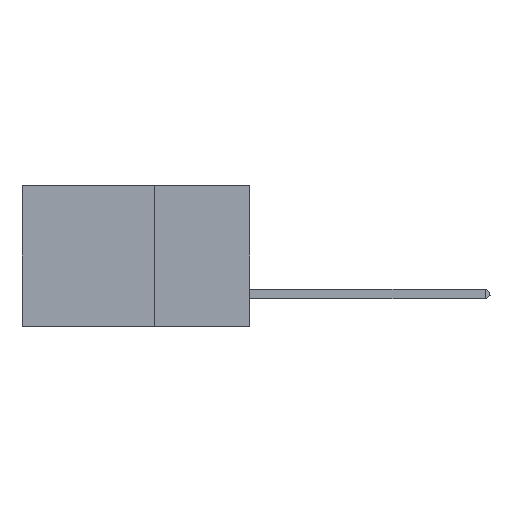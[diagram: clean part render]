
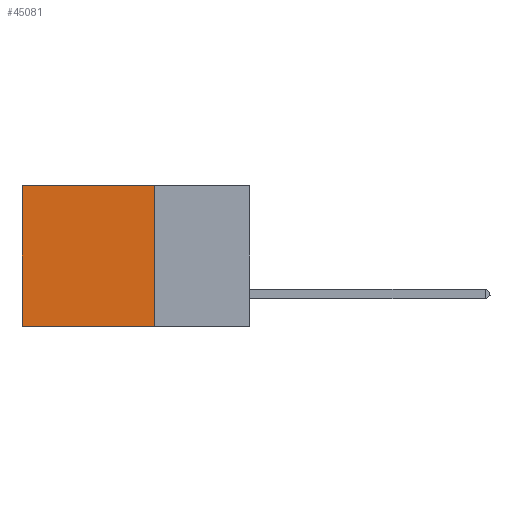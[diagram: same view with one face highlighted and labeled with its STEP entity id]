
A CAD part, left-side view. The second image highlights one B-rep face of the part: STEP entity #45081.
In plain terms, the highlighted planar face has unit normal (-1, 0, 0).
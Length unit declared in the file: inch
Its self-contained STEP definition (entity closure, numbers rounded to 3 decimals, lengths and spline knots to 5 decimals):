
#722 = LINE ( 'NONE', #14914, #33450 ) ;
#1972 = DIRECTION ( 'NONE',  ( 0., 0., -1. ) ) ;
#2355 = CARTESIAN_POINT ( 'NONE',  ( 0.2875, 0.25, -0.37 ) ) ;
#5395 = VECTOR ( 'NONE', #29505, 39.37008 ) ;
#6862 = CARTESIAN_POINT ( 'NONE',  ( 0.2875, 0.25, 0. ) ) ;
#7725 = DIRECTION ( 'NONE',  ( 0., 0., -1. ) ) ;
#8101 = LINE ( 'NONE', #22317, #5395 ) ;
#10496 = LINE ( 'NONE', #39095, #35112 ) ;
#10878 = AXIS2_PLACEMENT_3D ( 'NONE', #18262, #42696, #7725 ) ;
#14370 = DIRECTION ( 'NONE',  ( 0., 1., 0. ) ) ;
#14786 = DIRECTION ( 'NONE',  ( 0., 1., 0. ) ) ;
#14914 = CARTESIAN_POINT ( 'NONE',  ( 0.2875, 0.6, 0. ) ) ;
#18262 = CARTESIAN_POINT ( 'NONE',  ( 0.2875, 0.25, 0. ) ) ;
#18369 = EDGE_CURVE ( 'NONE', #37599, #29723, #10496, .T. ) ;
#18523 = ORIENTED_EDGE ( 'NONE', *, *, #36782, .T. ) ;
#19601 = EDGE_CURVE ( 'NONE', #42427, #36716, #27697, .T. ) ;
#21453 = PLANE ( 'NONE',  #10878 ) ;
#22317 = CARTESIAN_POINT ( 'NONE',  ( 0.2875, 0.25, 0. ) ) ;
#22323 = EDGE_LOOP ( 'NONE', ( #18523, #27617, #31021, #44815 ) ) ;
#27269 = FACE_OUTER_BOUND ( 'NONE', #22323, .T. ) ;
#27617 = ORIENTED_EDGE ( 'NONE', *, *, #18369, .F. ) ;
#27697 = LINE ( 'NONE', #32080, #41931 ) ;
#29505 = DIRECTION ( 'NONE',  ( 0., 0., -1. ) ) ;
#29723 = VERTEX_POINT ( 'NONE', #44958 ) ;
#31021 = ORIENTED_EDGE ( 'NONE', *, *, #33689, .F. ) ;
#32080 = CARTESIAN_POINT ( 'NONE',  ( 0.2875, 0.25, 0. ) ) ;
#33450 = VECTOR ( 'NONE', #1972, 39.37008 ) ;
#33689 = EDGE_CURVE ( 'NONE', #42427, #37599, #8101, .T. ) ;
#35112 = VECTOR ( 'NONE', #14786, 39.37008 ) ;
#36716 = VERTEX_POINT ( 'NONE', #38909 ) ;
#36782 = EDGE_CURVE ( 'NONE', #36716, #29723, #722, .T. ) ;
#37599 = VERTEX_POINT ( 'NONE', #2355 ) ;
#38909 = CARTESIAN_POINT ( 'NONE',  ( 0.2875, 0.6, 0. ) ) ;
#39095 = CARTESIAN_POINT ( 'NONE',  ( 0.2875, 0.25, -0.37 ) ) ;
#41931 = VECTOR ( 'NONE', #14370, 39.37008 ) ;
#42427 = VERTEX_POINT ( 'NONE', #6862 ) ;
#42696 = DIRECTION ( 'NONE',  ( 1., 0., 0. ) ) ;
#44815 = ORIENTED_EDGE ( 'NONE', *, *, #19601, .T. ) ;
#44958 = CARTESIAN_POINT ( 'NONE',  ( 0.2875, 0.6, -0.37 ) ) ;
#45081 = ADVANCED_FACE ( 'NONE', ( #27269 ), #21453, .F. ) ;
